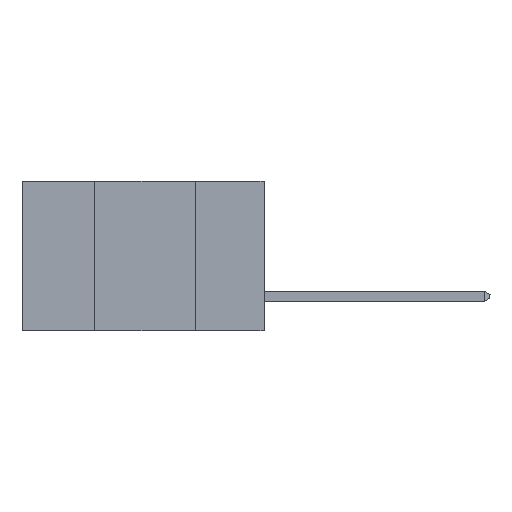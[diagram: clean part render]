
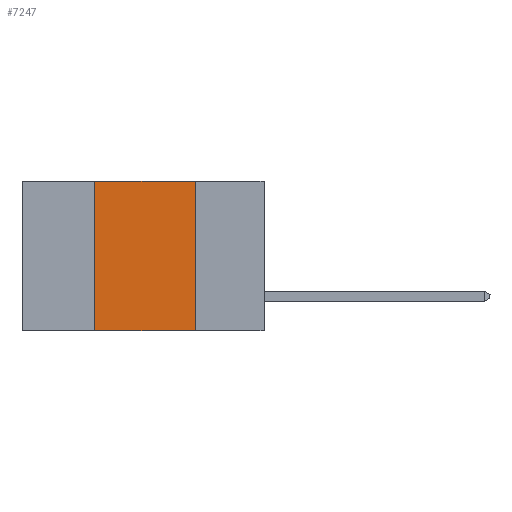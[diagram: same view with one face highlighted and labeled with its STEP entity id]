
A CAD part, left-side view. The second image highlights one B-rep face of the part: STEP entity #7247.
In plain terms, the highlighted planar face has unit normal (-1, 0, 0).
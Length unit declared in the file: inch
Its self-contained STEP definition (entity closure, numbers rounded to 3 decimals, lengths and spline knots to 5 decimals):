
#272 = VERTEX_POINT ( 'NONE', #4197 ) ;
#1140 = VECTOR ( 'NONE', #3723, 39.37008 ) ;
#1206 = PLANE ( 'NONE',  #6051 ) ;
#1485 = ORIENTED_EDGE ( 'NONE', *, *, #5940, .F. ) ;
#1871 = ORIENTED_EDGE ( 'NONE', *, *, #5916, .F. ) ;
#1997 = VERTEX_POINT ( 'NONE', #11785 ) ;
#2501 = VECTOR ( 'NONE', #4214, 39.37008 ) ;
#2587 = CARTESIAN_POINT ( 'NONE',  ( 0., 0.42, 0. ) ) ;
#3235 = CARTESIAN_POINT ( 'NONE',  ( 0., 0.6, -0.37 ) ) ;
#3304 = EDGE_CURVE ( 'NONE', #4433, #1997, #8821, .T. ) ;
#3353 = CARTESIAN_POINT ( 'NONE',  ( 0., 0.42, -0.37 ) ) ;
#3723 = DIRECTION ( 'NONE',  ( 0., 0., 1. ) ) ;
#3925 = EDGE_CURVE ( 'NONE', #7463, #272, #11850, .T. ) ;
#4197 = CARTESIAN_POINT ( 'NONE',  ( 0., 0.17, 0. ) ) ;
#4214 = DIRECTION ( 'NONE',  ( 0., -1., 0. ) ) ;
#4433 = VERTEX_POINT ( 'NONE', #3353 ) ;
#4445 = CARTESIAN_POINT ( 'NONE',  ( 0., 0.6, 0. ) ) ;
#4720 = ORIENTED_EDGE ( 'NONE', *, *, #3304, .T. ) ;
#4731 = DIRECTION ( 'NONE',  ( 0., 0., -1. ) ) ;
#5700 = VECTOR ( 'NONE', #7468, 39.37008 ) ;
#5916 = EDGE_CURVE ( 'NONE', #272, #1997, #10223, .T. ) ;
#5940 = EDGE_CURVE ( 'NONE', #4433, #7463, #9369, .T. ) ;
#6051 = AXIS2_PLACEMENT_3D ( 'NONE', #4445, #8827, #7779 ) ;
#6548 = CARTESIAN_POINT ( 'NONE',  ( 0., 0.6, 0. ) ) ;
#7247 = ADVANCED_FACE ( 'NONE', ( #13901 ), #1206, .F. ) ;
#7463 = VERTEX_POINT ( 'NONE', #2587 ) ;
#7468 = DIRECTION ( 'NONE',  ( 0., -1., 0. ) ) ;
#7779 = DIRECTION ( 'NONE',  ( 0., 0., -1. ) ) ;
#8821 = LINE ( 'NONE', #3235, #2501 ) ;
#8827 = DIRECTION ( 'NONE',  ( 1., 0., 0. ) ) ;
#9194 = CARTESIAN_POINT ( 'NONE',  ( 0., 0.42, 0. ) ) ;
#9369 = LINE ( 'NONE', #9194, #1140 ) ;
#10223 = LINE ( 'NONE', #11245, #13091 ) ;
#10740 = ORIENTED_EDGE ( 'NONE', *, *, #3925, .F. ) ;
#11245 = CARTESIAN_POINT ( 'NONE',  ( 0., 0.17, 0. ) ) ;
#11785 = CARTESIAN_POINT ( 'NONE',  ( 0., 0.17, -0.37 ) ) ;
#11850 = LINE ( 'NONE', #6548, #5700 ) ;
#12156 = EDGE_LOOP ( 'NONE', ( #1871, #10740, #1485, #4720 ) ) ;
#13091 = VECTOR ( 'NONE', #4731, 39.37008 ) ;
#13901 = FACE_OUTER_BOUND ( 'NONE', #12156, .T. ) ;
